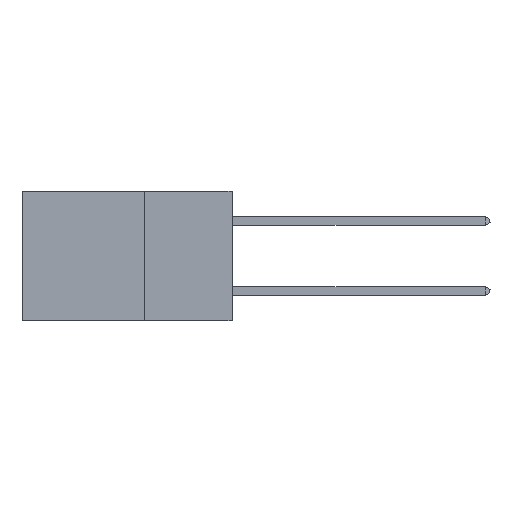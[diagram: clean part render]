
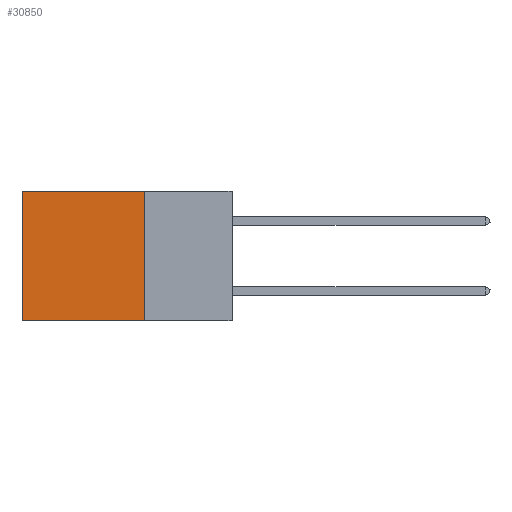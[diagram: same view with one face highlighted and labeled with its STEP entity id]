
A CAD part, left-side view. The second image highlights one B-rep face of the part: STEP entity #30850.
In plain terms, the highlighted planar face has unit normal (-1, 0, 0).
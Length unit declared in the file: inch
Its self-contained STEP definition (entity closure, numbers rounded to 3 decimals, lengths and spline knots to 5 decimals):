
#1064 = DIRECTION ( 'NONE',  ( 0., 1., 0. ) ) ;
#2291 = CARTESIAN_POINT ( 'NONE',  ( 0.2875, 0.25, -0.37 ) ) ;
#2675 = LINE ( 'NONE', #30948, #30339 ) ;
#5812 = CARTESIAN_POINT ( 'NONE',  ( 0.2875, 0.25, 0. ) ) ;
#6111 = ORIENTED_EDGE ( 'NONE', *, *, #28213, .T. ) ;
#6950 = DIRECTION ( 'NONE',  ( 0., 0., -1. ) ) ;
#7916 = EDGE_CURVE ( 'NONE', #29908, #12753, #2675, .T. ) ;
#8460 = ORIENTED_EDGE ( 'NONE', *, *, #7916, .F. ) ;
#9040 = AXIS2_PLACEMENT_3D ( 'NONE', #25292, #17745, #20419 ) ;
#9171 = CARTESIAN_POINT ( 'NONE',  ( 0.2875, 0.6, -0.37 ) ) ;
#9228 = VECTOR ( 'NONE', #14011, 39.37008 ) ;
#9648 = VECTOR ( 'NONE', #1064, 39.37008 ) ;
#11303 = EDGE_LOOP ( 'NONE', ( #16303, #32025, #8460, #6111 ) ) ;
#12753 = VERTEX_POINT ( 'NONE', #2291 ) ;
#12869 = DIRECTION ( 'NONE',  ( 0., 0., -1. ) ) ;
#14011 = DIRECTION ( 'NONE',  ( 0., 1., 0. ) ) ;
#14207 = CARTESIAN_POINT ( 'NONE',  ( 0.2875, 0.25, -0.37 ) ) ;
#14670 = EDGE_CURVE ( 'NONE', #21749, #23621, #33942, .T. ) ;
#15127 = LINE ( 'NONE', #14207, #9648 ) ;
#16303 = ORIENTED_EDGE ( 'NONE', *, *, #14670, .T. ) ;
#17627 = PLANE ( 'NONE',  #9040 ) ;
#17745 = DIRECTION ( 'NONE',  ( 1., 0., 0. ) ) ;
#20255 = CARTESIAN_POINT ( 'NONE',  ( 0.2875, 0.25, 0. ) ) ;
#20419 = DIRECTION ( 'NONE',  ( 0., 0., -1. ) ) ;
#21749 = VERTEX_POINT ( 'NONE', #22707 ) ;
#22707 = CARTESIAN_POINT ( 'NONE',  ( 0.2875, 0.6, 0. ) ) ;
#22996 = EDGE_CURVE ( 'NONE', #12753, #23621, #15127, .T. ) ;
#23621 = VERTEX_POINT ( 'NONE', #9171 ) ;
#23638 = CARTESIAN_POINT ( 'NONE',  ( 0.2875, 0.6, 0. ) ) ;
#25292 = CARTESIAN_POINT ( 'NONE',  ( 0.2875, 0.25, 0. ) ) ;
#28213 = EDGE_CURVE ( 'NONE', #29908, #21749, #30625, .T. ) ;
#29908 = VERTEX_POINT ( 'NONE', #20255 ) ;
#30044 = FACE_OUTER_BOUND ( 'NONE', #11303, .T. ) ;
#30339 = VECTOR ( 'NONE', #6950, 39.37008 ) ;
#30625 = LINE ( 'NONE', #5812, #9228 ) ;
#30850 = ADVANCED_FACE ( 'NONE', ( #30044 ), #17627, .F. ) ;
#30948 = CARTESIAN_POINT ( 'NONE',  ( 0.2875, 0.25, 0. ) ) ;
#32025 = ORIENTED_EDGE ( 'NONE', *, *, #22996, .F. ) ;
#32221 = VECTOR ( 'NONE', #12869, 39.37008 ) ;
#33942 = LINE ( 'NONE', #23638, #32221 ) ;
